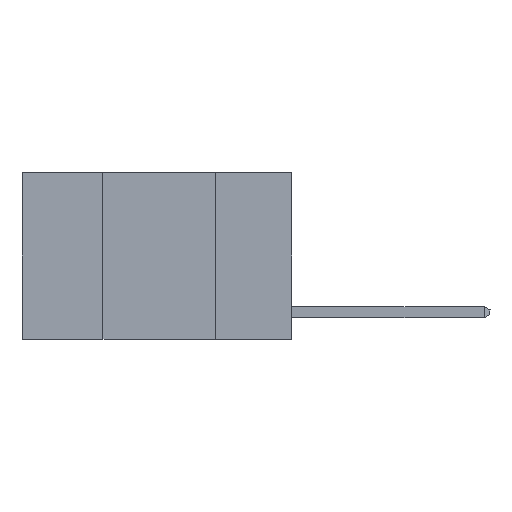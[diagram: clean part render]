
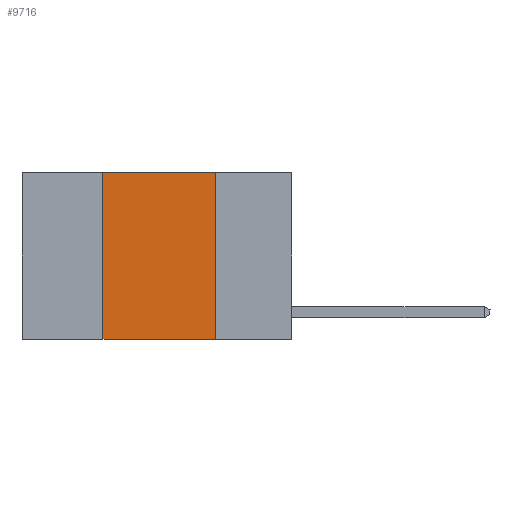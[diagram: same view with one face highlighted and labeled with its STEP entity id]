
A CAD part, left-side view. The second image highlights one B-rep face of the part: STEP entity #9716.
In plain terms, the highlighted planar face has unit normal (-1, 0, 0).
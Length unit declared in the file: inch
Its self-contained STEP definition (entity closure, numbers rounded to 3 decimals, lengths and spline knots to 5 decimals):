
#306 = PLANE ( 'NONE',  #21200 ) ;
#1454 = VERTEX_POINT ( 'NONE', #13186 ) ;
#3161 = DIRECTION ( 'NONE',  ( 0., -1., 0. ) ) ;
#3313 = CARTESIAN_POINT ( 'NONE',  ( 0., 0.6, 0. ) ) ;
#3558 = CARTESIAN_POINT ( 'NONE',  ( 0., 0.42, 0. ) ) ;
#4469 = CARTESIAN_POINT ( 'NONE',  ( 0., 0.17, 0. ) ) ;
#4543 = EDGE_CURVE ( 'NONE', #9617, #1454, #13028, .T. ) ;
#5518 = DIRECTION ( 'NONE',  ( 1., 0., 0. ) ) ;
#5742 = VERTEX_POINT ( 'NONE', #17417 ) ;
#5987 = ORIENTED_EDGE ( 'NONE', *, *, #8097, .F. ) ;
#6458 = EDGE_CURVE ( 'NONE', #5742, #21656, #8458, .T. ) ;
#7371 = ORIENTED_EDGE ( 'NONE', *, *, #4543, .F. ) ;
#7863 = DIRECTION ( 'NONE',  ( 0., 0., -1. ) ) ;
#8097 = EDGE_CURVE ( 'NONE', #5742, #9617, #8378, .T. ) ;
#8378 = LINE ( 'NONE', #10295, #11061 ) ;
#8458 = LINE ( 'NONE', #13520, #17410 ) ;
#9617 = VERTEX_POINT ( 'NONE', #3558 ) ;
#9716 = ADVANCED_FACE ( 'NONE', ( #20232 ), #306, .F. ) ;
#10295 = CARTESIAN_POINT ( 'NONE',  ( 0., 0.42, 0. ) ) ;
#10802 = DIRECTION ( 'NONE',  ( 0., 0., -1. ) ) ;
#11061 = VECTOR ( 'NONE', #15431, 39.37008 ) ;
#11295 = ORIENTED_EDGE ( 'NONE', *, *, #6458, .T. ) ;
#12864 = EDGE_CURVE ( 'NONE', #1454, #21656, #21532, .T. ) ;
#13028 = LINE ( 'NONE', #3313, #17110 ) ;
#13186 = CARTESIAN_POINT ( 'NONE',  ( 0., 0.17, 0. ) ) ;
#13520 = CARTESIAN_POINT ( 'NONE',  ( 0., 0.6, -0.37 ) ) ;
#13755 = DIRECTION ( 'NONE',  ( 0., -1., 0. ) ) ;
#14242 = VECTOR ( 'NONE', #7863, 39.37008 ) ;
#15431 = DIRECTION ( 'NONE',  ( 0., 0., 1. ) ) ;
#15926 = CARTESIAN_POINT ( 'NONE',  ( 0., 0.17, -0.37 ) ) ;
#17110 = VECTOR ( 'NONE', #13755, 39.37008 ) ;
#17410 = VECTOR ( 'NONE', #3161, 39.37008 ) ;
#17417 = CARTESIAN_POINT ( 'NONE',  ( 0., 0.42, -0.37 ) ) ;
#17606 = ORIENTED_EDGE ( 'NONE', *, *, #12864, .F. ) ;
#18286 = EDGE_LOOP ( 'NONE', ( #17606, #7371, #5987, #11295 ) ) ;
#19369 = CARTESIAN_POINT ( 'NONE',  ( 0., 0.6, 0. ) ) ;
#20232 = FACE_OUTER_BOUND ( 'NONE', #18286, .T. ) ;
#21200 = AXIS2_PLACEMENT_3D ( 'NONE', #19369, #5518, #10802 ) ;
#21532 = LINE ( 'NONE', #4469, #14242 ) ;
#21656 = VERTEX_POINT ( 'NONE', #15926 ) ;
